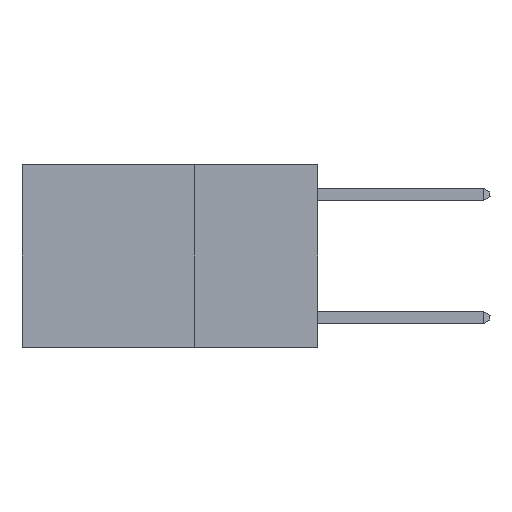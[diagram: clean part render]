
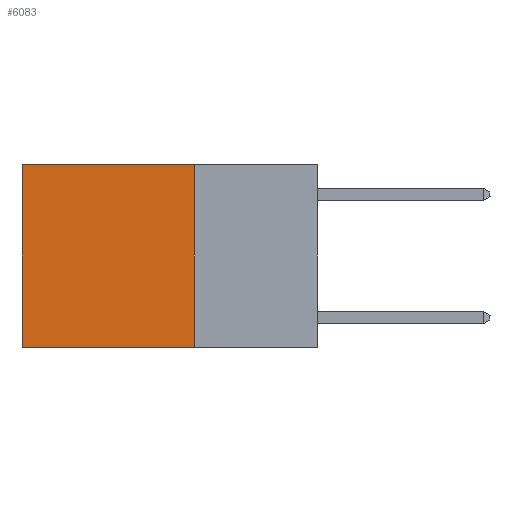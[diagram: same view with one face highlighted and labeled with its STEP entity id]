
A CAD part, left-side view. The second image highlights one B-rep face of the part: STEP entity #6083.
In plain terms, the highlighted planar face has unit normal (-1, 0, 0).
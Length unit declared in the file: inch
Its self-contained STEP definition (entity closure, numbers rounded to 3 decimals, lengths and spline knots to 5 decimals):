
#321 = ORIENTED_EDGE ( 'NONE', *, *, #3328, .T. ) ;
#359 = VECTOR ( 'NONE', #9108, 39.37008 ) ;
#438 = FACE_OUTER_BOUND ( 'NONE', #4287, .T. ) ;
#908 = EDGE_CURVE ( 'NONE', #9004, #6638, #4526, .T. ) ;
#2109 = DIRECTION ( 'NONE',  ( 0., 0., -1. ) ) ;
#2156 = EDGE_CURVE ( 'NONE', #6638, #2653, #9892, .T. ) ;
#2378 = AXIS2_PLACEMENT_3D ( 'NONE', #6831, #10029, #7924 ) ;
#2653 = VERTEX_POINT ( 'NONE', #10074 ) ;
#2832 = ORIENTED_EDGE ( 'NONE', *, *, #2156, .F. ) ;
#2890 = CARTESIAN_POINT ( 'NONE',  ( 0.2625, 0.25, -0.37 ) ) ;
#3328 = EDGE_CURVE ( 'NONE', #9004, #10014, #6546, .T. ) ;
#3653 = PLANE ( 'NONE',  #2378 ) ;
#4287 = EDGE_LOOP ( 'NONE', ( #8751, #2832, #8755, #321 ) ) ;
#4526 = LINE ( 'NONE', #6041, #8921 ) ;
#4890 = CARTESIAN_POINT ( 'NONE',  ( 0.2625, 0.25, -0.37 ) ) ;
#5188 = LINE ( 'NONE', #6807, #6860 ) ;
#5657 = CARTESIAN_POINT ( 'NONE',  ( 0.2625, 0.25, 0. ) ) ;
#6041 = CARTESIAN_POINT ( 'NONE',  ( 0.2625, 0.25, 0. ) ) ;
#6083 = ADVANCED_FACE ( 'NONE', ( #438 ), #3653, .F. ) ;
#6546 = LINE ( 'NONE', #6698, #9635 ) ;
#6638 = VERTEX_POINT ( 'NONE', #4890 ) ;
#6698 = CARTESIAN_POINT ( 'NONE',  ( 0.2625, 0.25, 0. ) ) ;
#6807 = CARTESIAN_POINT ( 'NONE',  ( 0.2625, 0.6, 0. ) ) ;
#6831 = CARTESIAN_POINT ( 'NONE',  ( 0.2625, 0.25, 0. ) ) ;
#6860 = VECTOR ( 'NONE', #8365, 39.37008 ) ;
#7418 = DIRECTION ( 'NONE',  ( 0., 1., 0. ) ) ;
#7924 = DIRECTION ( 'NONE',  ( 0., 0., -1. ) ) ;
#8136 = EDGE_CURVE ( 'NONE', #10014, #2653, #5188, .T. ) ;
#8365 = DIRECTION ( 'NONE',  ( 0., 0., -1. ) ) ;
#8405 = CARTESIAN_POINT ( 'NONE',  ( 0.2625, 0.6, 0. ) ) ;
#8751 = ORIENTED_EDGE ( 'NONE', *, *, #8136, .T. ) ;
#8755 = ORIENTED_EDGE ( 'NONE', *, *, #908, .F. ) ;
#8921 = VECTOR ( 'NONE', #2109, 39.37008 ) ;
#9004 = VERTEX_POINT ( 'NONE', #5657 ) ;
#9108 = DIRECTION ( 'NONE',  ( 0., 1., 0. ) ) ;
#9635 = VECTOR ( 'NONE', #7418, 39.37008 ) ;
#9892 = LINE ( 'NONE', #2890, #359 ) ;
#10014 = VERTEX_POINT ( 'NONE', #8405 ) ;
#10029 = DIRECTION ( 'NONE',  ( 1., 0., 0. ) ) ;
#10074 = CARTESIAN_POINT ( 'NONE',  ( 0.2625, 0.6, -0.37 ) ) ;
